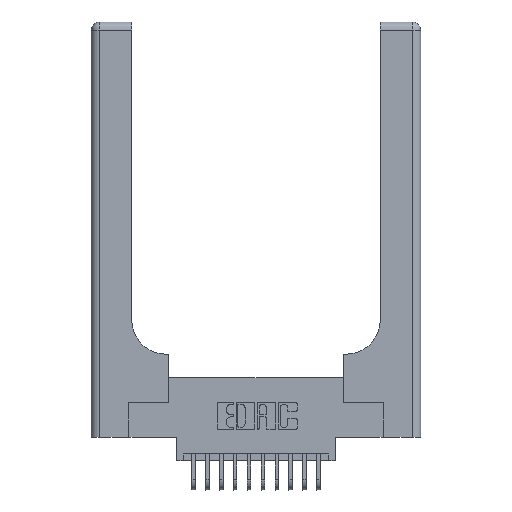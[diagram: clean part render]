
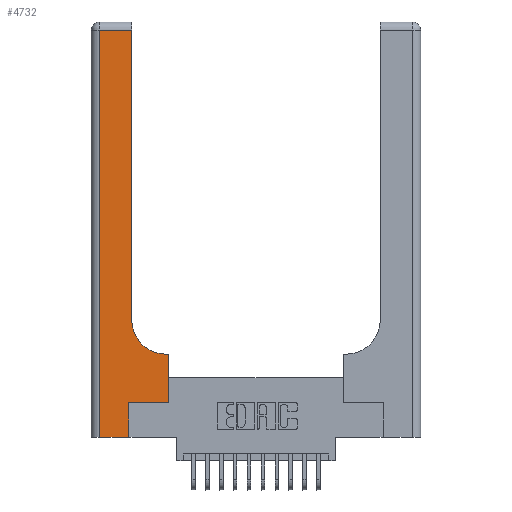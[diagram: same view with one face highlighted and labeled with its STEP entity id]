
A CAD part, top view. The second image highlights one B-rep face of the part: STEP entity #4732.
In plain terms, the highlighted planar face has unit normal (0, 0, 1).
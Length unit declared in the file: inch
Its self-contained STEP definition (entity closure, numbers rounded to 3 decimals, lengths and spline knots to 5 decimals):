
#116 = AXIS2_PLACEMENT_3D ( 'NONE', #15504, #18335, #9810 ) ;
#453 = ORIENTED_EDGE ( 'NONE', *, *, #512, .T. ) ;
#512 = EDGE_CURVE ( 'NONE', #12440, #11681, #6418, .T. ) ;
#524 = DIRECTION ( 'NONE',  ( -1., 0., 0. ) ) ;
#901 = CARTESIAN_POINT ( 'NONE',  ( 0.269, 0., 0.37 ) ) ;
#1083 = CARTESIAN_POINT ( 'NONE',  ( 0., 2.94, 0.37 ) ) ;
#1314 = EDGE_CURVE ( 'NONE', #7096, #17783, #10160, .T. ) ;
#1490 = VECTOR ( 'NONE', #7038, 39.37008 ) ;
#1495 = EDGE_CURVE ( 'NONE', #2396, #2050, #4156, .T. ) ;
#1987 = CARTESIAN_POINT ( 'NONE',  ( 0.2915, 2.94, 0.37 ) ) ;
#2050 = VERTEX_POINT ( 'NONE', #901 ) ;
#2396 = VERTEX_POINT ( 'NONE', #8413 ) ;
#2423 = CARTESIAN_POINT ( 'NONE',  ( 0.2915, 3., 0.37 ) ) ;
#2666 = EDGE_CURVE ( 'NONE', #7408, #3187, #11027, .T. ) ;
#2719 = VECTOR ( 'NONE', #9972, 39.37008 ) ;
#3187 = VERTEX_POINT ( 'NONE', #19025 ) ;
#3405 = CARTESIAN_POINT ( 'NONE',  ( 0.5585, 0.25, 0.37 ) ) ;
#3659 = LINE ( 'NONE', #15761, #11234 ) ;
#3912 = VECTOR ( 'NONE', #524, 39.37008 ) ;
#4133 = CARTESIAN_POINT ( 'NONE',  ( 0.269, 0.25, 0.37 ) ) ;
#4156 = LINE ( 'NONE', #5793, #14629 ) ;
#4237 = ORIENTED_EDGE ( 'NONE', *, *, #16504, .T. ) ;
#4732 = ADVANCED_FACE ( 'NONE', ( #9573 ), #9739, .F. ) ;
#5656 = DIRECTION ( 'NONE',  ( 1., 0., 0. ) ) ;
#5793 = CARTESIAN_POINT ( 'NONE',  ( 0., 0., 0.37 ) ) ;
#6109 = ORIENTED_EDGE ( 'NONE', *, *, #1314, .T. ) ;
#6418 = CIRCLE ( 'NONE', #17891, 0.25 ) ;
#6706 = EDGE_LOOP ( 'NONE', ( #16469, #8537, #14154, #14553, #13142, #6109, #9191, #4237, #453 ) ) ;
#6802 = LINE ( 'NONE', #15667, #2719 ) ;
#6822 = CARTESIAN_POINT ( 'NONE',  ( 0.269, 0.25, 0.37 ) ) ;
#6823 = CARTESIAN_POINT ( 'NONE',  ( 0.5585, 0.25, 0.37 ) ) ;
#7038 = DIRECTION ( 'NONE',  ( 0., 1., 0. ) ) ;
#7096 = VERTEX_POINT ( 'NONE', #4133 ) ;
#7319 = CARTESIAN_POINT ( 'NONE',  ( 0.5585, 0.6, 0.37 ) ) ;
#7408 = VERTEX_POINT ( 'NONE', #1987 ) ;
#7637 = EDGE_CURVE ( 'NONE', #2050, #7096, #15016, .T. ) ;
#8358 = DIRECTION ( 'NONE',  ( 0., 1., 0. ) ) ;
#8413 = CARTESIAN_POINT ( 'NONE',  ( 0.06, 0., 0.37 ) ) ;
#8537 = ORIENTED_EDGE ( 'NONE', *, *, #2666, .T. ) ;
#9126 = LINE ( 'NONE', #2423, #1490 ) ;
#9191 = ORIENTED_EDGE ( 'NONE', *, *, #19000, .T. ) ;
#9383 = LINE ( 'NONE', #6823, #12816 ) ;
#9573 = FACE_OUTER_BOUND ( 'NONE', #6706, .T. ) ;
#9701 = VECTOR ( 'NONE', #12493, 39.37008 ) ;
#9739 = PLANE ( 'NONE',  #116 ) ;
#9810 = DIRECTION ( 'NONE',  ( -1., 0., 0. ) ) ;
#9972 = DIRECTION ( 'NONE',  ( 0., -1., 0. ) ) ;
#10013 = CARTESIAN_POINT ( 'NONE',  ( 0.269, 0., 0.37 ) ) ;
#10160 = LINE ( 'NONE', #6822, #9701 ) ;
#11027 = LINE ( 'NONE', #1083, #3912 ) ;
#11234 = VECTOR ( 'NONE', #17186, 39.37008 ) ;
#11397 = DIRECTION ( 'NONE',  ( 1., 0., 0. ) ) ;
#11414 = DIRECTION ( 'NONE',  ( 0., 0., -1. ) ) ;
#11475 = DIRECTION ( 'NONE',  ( 0., 1., 0. ) ) ;
#11484 = CARTESIAN_POINT ( 'NONE',  ( 0.5415, 0.6, 0.37 ) ) ;
#11681 = VERTEX_POINT ( 'NONE', #17099 ) ;
#12440 = VERTEX_POINT ( 'NONE', #11484 ) ;
#12493 = DIRECTION ( 'NONE',  ( 1., 0., 0. ) ) ;
#12816 = VECTOR ( 'NONE', #8358, 39.37008 ) ;
#13142 = ORIENTED_EDGE ( 'NONE', *, *, #7637, .T. ) ;
#13916 = CARTESIAN_POINT ( 'NONE',  ( 0.5415, 0.85, 0.37 ) ) ;
#14154 = ORIENTED_EDGE ( 'NONE', *, *, #16985, .T. ) ;
#14553 = ORIENTED_EDGE ( 'NONE', *, *, #1495, .T. ) ;
#14580 = VECTOR ( 'NONE', #11475, 39.37008 ) ;
#14629 = VECTOR ( 'NONE', #5656, 39.37008 ) ;
#15016 = LINE ( 'NONE', #10013, #14580 ) ;
#15301 = VERTEX_POINT ( 'NONE', #7319 ) ;
#15504 = CARTESIAN_POINT ( 'NONE',  ( 0., 3., 0.37 ) ) ;
#15667 = CARTESIAN_POINT ( 'NONE',  ( 0.06, 3., 0.37 ) ) ;
#15761 = CARTESIAN_POINT ( 'NONE',  ( 0.2915, 0.6, 0.37 ) ) ;
#16469 = ORIENTED_EDGE ( 'NONE', *, *, #18513, .T. ) ;
#16504 = EDGE_CURVE ( 'NONE', #15301, #12440, #3659, .T. ) ;
#16985 = EDGE_CURVE ( 'NONE', #3187, #2396, #6802, .T. ) ;
#17099 = CARTESIAN_POINT ( 'NONE',  ( 0.2915, 0.85, 0.37 ) ) ;
#17186 = DIRECTION ( 'NONE',  ( -1., 0., 0. ) ) ;
#17783 = VERTEX_POINT ( 'NONE', #3405 ) ;
#17891 = AXIS2_PLACEMENT_3D ( 'NONE', #13916, #11414, #11397 ) ;
#18335 = DIRECTION ( 'NONE',  ( 0., 0., -1. ) ) ;
#18513 = EDGE_CURVE ( 'NONE', #11681, #7408, #9126, .T. ) ;
#19000 = EDGE_CURVE ( 'NONE', #17783, #15301, #9383, .T. ) ;
#19025 = CARTESIAN_POINT ( 'NONE',  ( 0.06, 2.94, 0.37 ) ) ;
